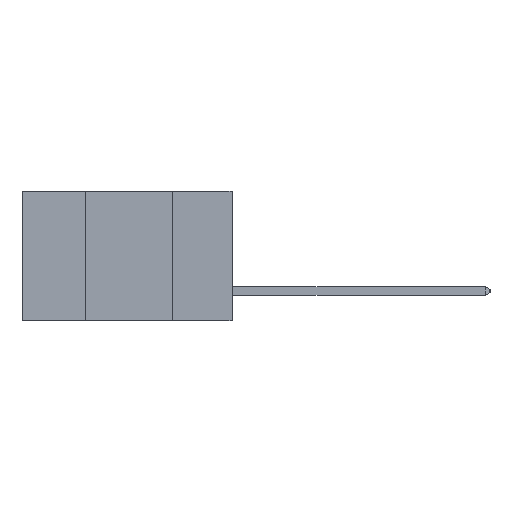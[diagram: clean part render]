
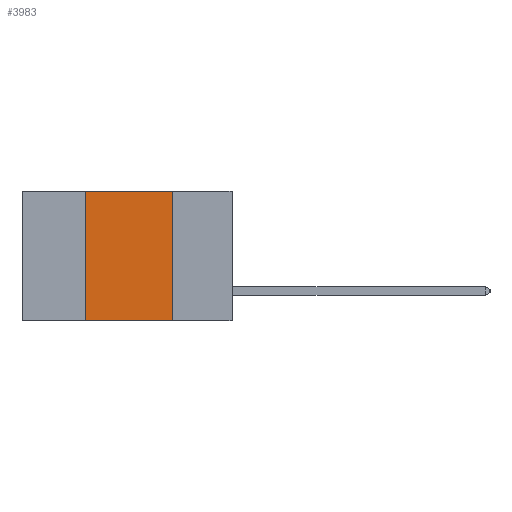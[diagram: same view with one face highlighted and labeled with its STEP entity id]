
A CAD part, left-side view. The second image highlights one B-rep face of the part: STEP entity #3983.
In plain terms, the highlighted planar face has unit normal (-1, 0, 0).
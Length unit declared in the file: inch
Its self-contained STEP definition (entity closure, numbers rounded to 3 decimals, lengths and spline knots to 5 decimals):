
#449 = FACE_OUTER_BOUND ( 'NONE', #11458, .T. ) ;
#2067 = CARTESIAN_POINT ( 'NONE',  ( 0., 0.6, 0. ) ) ;
#2075 = VERTEX_POINT ( 'NONE', #11222 ) ;
#2543 = VECTOR ( 'NONE', #11180, 39.37008 ) ;
#3433 = CARTESIAN_POINT ( 'NONE',  ( 0., 0.6, 0. ) ) ;
#3983 = ADVANCED_FACE ( 'NONE', ( #449 ), #4596, .F. ) ;
#4448 = VERTEX_POINT ( 'NONE', #9091 ) ;
#4596 = PLANE ( 'NONE',  #8875 ) ;
#5261 = CARTESIAN_POINT ( 'NONE',  ( 0., 0.42, 0. ) ) ;
#5356 = EDGE_CURVE ( 'NONE', #2075, #7732, #15518, .T. ) ;
#5655 = CARTESIAN_POINT ( 'NONE',  ( 0., 0.6, -0.37 ) ) ;
#5804 = DIRECTION ( 'NONE',  ( 0., 0., -1. ) ) ;
#5930 = DIRECTION ( 'NONE',  ( 0., -1., 0. ) ) ;
#6075 = VECTOR ( 'NONE', #5930, 39.37008 ) ;
#6460 = DIRECTION ( 'NONE',  ( 0., 0., 1. ) ) ;
#7732 = VERTEX_POINT ( 'NONE', #14779 ) ;
#7839 = CARTESIAN_POINT ( 'NONE',  ( 0., 0.42, -0.37 ) ) ;
#8735 = ORIENTED_EDGE ( 'NONE', *, *, #10935, .T. ) ;
#8875 = AXIS2_PLACEMENT_3D ( 'NONE', #2067, #12910, #5804 ) ;
#9091 = CARTESIAN_POINT ( 'NONE',  ( 0., 0.17, -0.37 ) ) ;
#9290 = ORIENTED_EDGE ( 'NONE', *, *, #5356, .F. ) ;
#9672 = VECTOR ( 'NONE', #12766, 39.37008 ) ;
#10935 = EDGE_CURVE ( 'NONE', #12625, #4448, #12787, .T. ) ;
#11180 = DIRECTION ( 'NONE',  ( 0., 0., -1. ) ) ;
#11222 = CARTESIAN_POINT ( 'NONE',  ( 0., 0.42, 0. ) ) ;
#11458 = EDGE_LOOP ( 'NONE', ( #12074, #9290, #12433, #8735 ) ) ;
#12074 = ORIENTED_EDGE ( 'NONE', *, *, #14865, .F. ) ;
#12156 = LINE ( 'NONE', #13541, #2543 ) ;
#12211 = LINE ( 'NONE', #5261, #14592 ) ;
#12433 = ORIENTED_EDGE ( 'NONE', *, *, #12503, .F. ) ;
#12503 = EDGE_CURVE ( 'NONE', #12625, #2075, #12211, .T. ) ;
#12625 = VERTEX_POINT ( 'NONE', #7839 ) ;
#12766 = DIRECTION ( 'NONE',  ( 0., -1., 0. ) ) ;
#12787 = LINE ( 'NONE', #5655, #9672 ) ;
#12910 = DIRECTION ( 'NONE',  ( 1., 0., 0. ) ) ;
#13541 = CARTESIAN_POINT ( 'NONE',  ( 0., 0.17, 0. ) ) ;
#14592 = VECTOR ( 'NONE', #6460, 39.37008 ) ;
#14779 = CARTESIAN_POINT ( 'NONE',  ( 0., 0.17, 0. ) ) ;
#14865 = EDGE_CURVE ( 'NONE', #7732, #4448, #12156, .T. ) ;
#15518 = LINE ( 'NONE', #3433, #6075 ) ;
